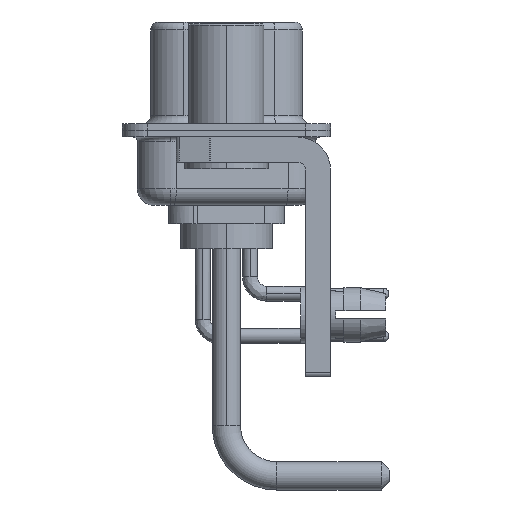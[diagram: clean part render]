
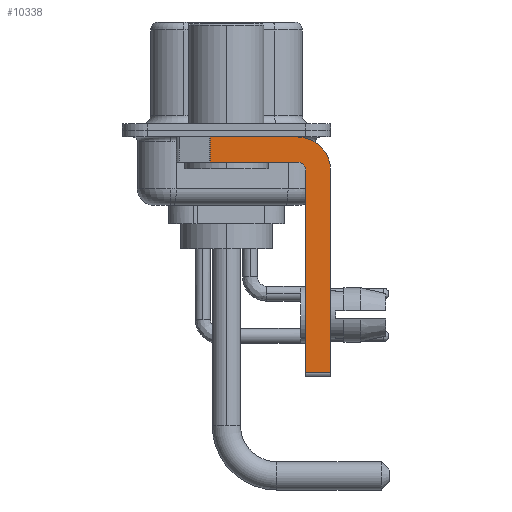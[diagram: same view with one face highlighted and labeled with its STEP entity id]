
A CAD part, left-side view. The second image highlights one B-rep face of the part: STEP entity #10338.
In plain terms, the highlighted planar face has unit normal (-1, 0, 0).
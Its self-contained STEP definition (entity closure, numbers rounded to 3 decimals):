
#765 = LINE ( 'NONE', #27034, #9288 ) ;
#1929 = LINE ( 'NONE', #21220, #14111 ) ;
#3300 = VECTOR ( 'NONE', #11562, 1000. ) ;
#4350 = CIRCLE ( 'NONE', #22199, 0.5 ) ;
#4723 = LINE ( 'NONE', #7129, #24686 ) ;
#5209 = AXIS2_PLACEMENT_3D ( 'NONE', #16328, #26009, #30621 ) ;
#5504 = DIRECTION ( 'NONE',  ( 0., 0., -1. ) ) ;
#5712 = VERTEX_POINT ( 'NONE', #15617 ) ;
#5991 = EDGE_CURVE ( 'NONE', #25909, #26566, #4723, .T. ) ;
#6754 = VERTEX_POINT ( 'NONE', #9857 ) ;
#6884 = LINE ( 'NONE', #9602, #11849 ) ;
#7129 = CARTESIAN_POINT ( 'NONE',  ( -2.9, 3., -0.4 ) ) ;
#8263 = DIRECTION ( 'NONE',  ( 0., 0., 1. ) ) ;
#9288 = VECTOR ( 'NONE', #20053, 1000. ) ;
#9310 = CARTESIAN_POINT ( 'NONE',  ( -2.9, -4.75, -14.55 ) ) ;
#9417 = CARTESIAN_POINT ( 'NONE',  ( -2.9, 0.978, -0.4 ) ) ;
#9602 = CARTESIAN_POINT ( 'NONE',  ( -2.9, -4.75, -14.8 ) ) ;
#9857 = CARTESIAN_POINT ( 'NONE',  ( -2.9, -6.25, -14.55 ) ) ;
#9979 = EDGE_CURVE ( 'NONE', #5712, #6754, #765, .T. ) ;
#10338 = ADVANCED_FACE ( 'NONE', ( #24140 ), #20983, .F. ) ;
#10340 = AXIS2_PLACEMENT_3D ( 'NONE', #12373, #29710, #5504 ) ;
#11295 = ORIENTED_EDGE ( 'NONE', *, *, #9979, .F. ) ;
#11562 = DIRECTION ( 'NONE',  ( 0., 0., -1. ) ) ;
#11849 = VECTOR ( 'NONE', #14556, 1000. ) ;
#11971 = EDGE_CURVE ( 'NONE', #20149, #6754, #21487, .T. ) ;
#12373 = CARTESIAN_POINT ( 'NONE',  ( -2.9, -4.25, -2.4 ) ) ;
#13899 = DIRECTION ( 'NONE',  ( 0., 1., 0. ) ) ;
#14111 = VECTOR ( 'NONE', #13899, 1000. ) ;
#14155 = CARTESIAN_POINT ( 'NONE',  ( -2.9, -4.75, -2.4 ) ) ;
#14523 = VERTEX_POINT ( 'NONE', #17263 ) ;
#14556 = DIRECTION ( 'NONE',  ( 0., 0., 1. ) ) ;
#14841 = CARTESIAN_POINT ( 'NONE',  ( -2.9, -4.25, -1.9 ) ) ;
#15297 = ORIENTED_EDGE ( 'NONE', *, *, #31366, .F. ) ;
#15538 = ORIENTED_EDGE ( 'NONE', *, *, #24055, .F. ) ;
#15617 = CARTESIAN_POINT ( 'NONE',  ( -2.9, -6.25, -2.4 ) ) ;
#16328 = CARTESIAN_POINT ( 'NONE',  ( -2.9, -4.25, -2.4 ) ) ;
#16869 = DIRECTION ( 'NONE',  ( 0., -1., 0. ) ) ;
#16896 = ORIENTED_EDGE ( 'NONE', *, *, #21045, .T. ) ;
#17263 = CARTESIAN_POINT ( 'NONE',  ( -2.9, 0.978, -1.9 ) ) ;
#17654 = ORIENTED_EDGE ( 'NONE', *, *, #5991, .F. ) ;
#18001 = CARTESIAN_POINT ( 'NONE',  ( -2.9, -4.25, -2.4 ) ) ;
#18328 = DIRECTION ( 'NONE',  ( -1., 0., 0. ) ) ;
#18857 = EDGE_CURVE ( 'NONE', #20149, #19699, #6884, .T. ) ;
#19117 = CARTESIAN_POINT ( 'NONE',  ( -2.9, -4.25, -14.55 ) ) ;
#19570 = ORIENTED_EDGE ( 'NONE', *, *, #18857, .F. ) ;
#19633 = CARTESIAN_POINT ( 'NONE',  ( -2.9, -4.25, -0.4 ) ) ;
#19699 = VERTEX_POINT ( 'NONE', #14155 ) ;
#20053 = DIRECTION ( 'NONE',  ( 0., 0., -1. ) ) ;
#20149 = VERTEX_POINT ( 'NONE', #9310 ) ;
#20983 = PLANE ( 'NONE',  #10340 ) ;
#21045 = EDGE_CURVE ( 'NONE', #25909, #14523, #23801, .T. ) ;
#21220 = CARTESIAN_POINT ( 'NONE',  ( -2.9, -4.25, -1.9 ) ) ;
#21487 = LINE ( 'NONE', #19117, #22118 ) ;
#22118 = VECTOR ( 'NONE', #28487, 1000. ) ;
#22199 = AXIS2_PLACEMENT_3D ( 'NONE', #18001, #18328, #8263 ) ;
#22604 = ORIENTED_EDGE ( 'NONE', *, *, #11971, .T. ) ;
#23334 = CARTESIAN_POINT ( 'NONE',  ( -2.9, 0.978, -1.9 ) ) ;
#23801 = LINE ( 'NONE', #23334, #3300 ) ;
#24040 = CIRCLE ( 'NONE', #5209, 2. ) ;
#24055 = EDGE_CURVE ( 'NONE', #26566, #5712, #24040, .T. ) ;
#24140 = FACE_OUTER_BOUND ( 'NONE', #24701, .T. ) ;
#24686 = VECTOR ( 'NONE', #16869, 1000. ) ;
#24701 = EDGE_LOOP ( 'NONE', ( #17654, #16896, #15297, #30900, #19570, #22604, #11295, #15538 ) ) ;
#25909 = VERTEX_POINT ( 'NONE', #9417 ) ;
#25994 = VERTEX_POINT ( 'NONE', #14841 ) ;
#26009 = DIRECTION ( 'NONE',  ( 1., 0., 0. ) ) ;
#26566 = VERTEX_POINT ( 'NONE', #19633 ) ;
#27034 = CARTESIAN_POINT ( 'NONE',  ( -2.9, -6.25, -2.4 ) ) ;
#28448 = EDGE_CURVE ( 'NONE', #19699, #25994, #4350, .T. ) ;
#28487 = DIRECTION ( 'NONE',  ( 0., -1., 0. ) ) ;
#29710 = DIRECTION ( 'NONE',  ( 1., 0., 0. ) ) ;
#30621 = DIRECTION ( 'NONE',  ( 0., 0., -1. ) ) ;
#30900 = ORIENTED_EDGE ( 'NONE', *, *, #28448, .F. ) ;
#31366 = EDGE_CURVE ( 'NONE', #25994, #14523, #1929, .T. ) ;
